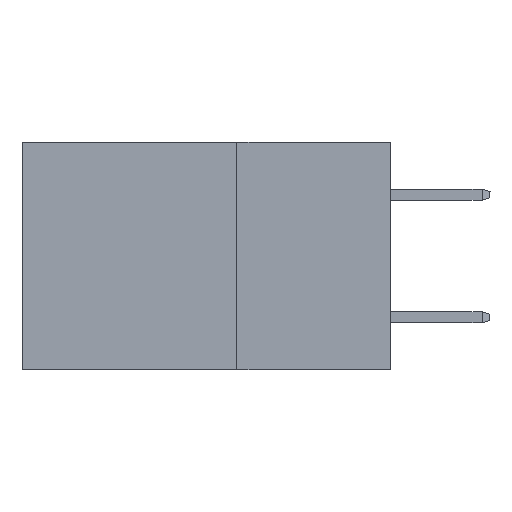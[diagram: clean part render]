
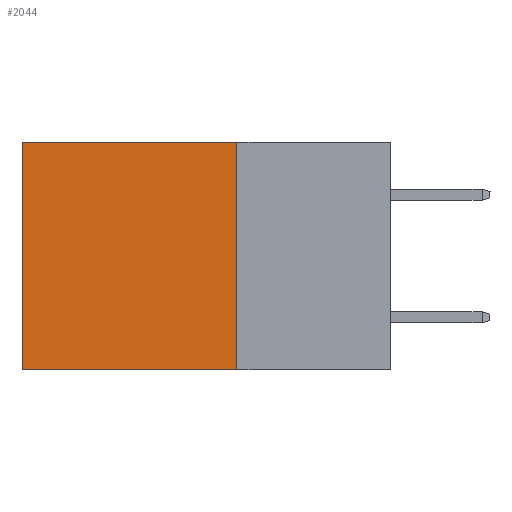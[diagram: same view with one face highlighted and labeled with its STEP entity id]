
A CAD part, left-side view. The second image highlights one B-rep face of the part: STEP entity #2044.
In plain terms, the highlighted planar face has unit normal (-1, 0, 0).
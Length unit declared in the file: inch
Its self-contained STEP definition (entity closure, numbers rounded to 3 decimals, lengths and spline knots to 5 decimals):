
#1630 = DIRECTION ( 'NONE',  ( 0., 1., 0. ) ) ;
#2005 = FACE_OUTER_BOUND ( 'NONE', #10825, .T. ) ;
#2044 = ADVANCED_FACE ( 'NONE', ( #2005 ), #17550, .F. ) ;
#2303 = VECTOR ( 'NONE', #1630, 39.37008 ) ;
#6398 = VECTOR ( 'NONE', #15519, 39.37008 ) ;
#6489 = CARTESIAN_POINT ( 'NONE',  ( 0.2875, 0.6, 0. ) ) ;
#6581 = LINE ( 'NONE', #12437, #2303 ) ;
#6946 = LINE ( 'NONE', #11987, #6398 ) ;
#6952 = DIRECTION ( 'NONE',  ( 0., 0., -1. ) ) ;
#10624 = ORIENTED_EDGE ( 'NONE', *, *, #14713, .T. ) ;
#10825 = EDGE_LOOP ( 'NONE', ( #21320, #17972, #13858, #10624 ) ) ;
#11648 = VECTOR ( 'NONE', #20529, 39.37008 ) ;
#11987 = CARTESIAN_POINT ( 'NONE',  ( 0.2875, 0.25, 0. ) ) ;
#12207 = LINE ( 'NONE', #18798, #11648 ) ;
#12398 = VERTEX_POINT ( 'NONE', #18010 ) ;
#12437 = CARTESIAN_POINT ( 'NONE',  ( 0.2875, 0.25, -0.37 ) ) ;
#12933 = DIRECTION ( 'NONE',  ( 0., 0., -1. ) ) ;
#13021 = LINE ( 'NONE', #21703, #21279 ) ;
#13337 = CARTESIAN_POINT ( 'NONE',  ( 0.2875, 0.25, 0. ) ) ;
#13858 = ORIENTED_EDGE ( 'NONE', *, *, #18443, .F. ) ;
#14713 = EDGE_CURVE ( 'NONE', #17749, #22465, #6946, .T. ) ;
#15519 = DIRECTION ( 'NONE',  ( 0., 1., 0. ) ) ;
#15844 = CARTESIAN_POINT ( 'NONE',  ( 0.2875, 0.25, 0. ) ) ;
#16215 = EDGE_CURVE ( 'NONE', #22465, #12398, #13021, .T. ) ;
#16424 = CARTESIAN_POINT ( 'NONE',  ( 0.2875, 0.25, -0.37 ) ) ;
#16731 = EDGE_CURVE ( 'NONE', #18204, #12398, #6581, .T. ) ;
#17550 = PLANE ( 'NONE',  #21333 ) ;
#17621 = DIRECTION ( 'NONE',  ( 1., 0., 0. ) ) ;
#17749 = VERTEX_POINT ( 'NONE', #13337 ) ;
#17972 = ORIENTED_EDGE ( 'NONE', *, *, #16731, .F. ) ;
#18010 = CARTESIAN_POINT ( 'NONE',  ( 0.2875, 0.6, -0.37 ) ) ;
#18204 = VERTEX_POINT ( 'NONE', #16424 ) ;
#18443 = EDGE_CURVE ( 'NONE', #17749, #18204, #12207, .T. ) ;
#18798 = CARTESIAN_POINT ( 'NONE',  ( 0.2875, 0.25, 0. ) ) ;
#20529 = DIRECTION ( 'NONE',  ( 0., 0., -1. ) ) ;
#21279 = VECTOR ( 'NONE', #12933, 39.37008 ) ;
#21320 = ORIENTED_EDGE ( 'NONE', *, *, #16215, .T. ) ;
#21333 = AXIS2_PLACEMENT_3D ( 'NONE', #15844, #17621, #6952 ) ;
#21703 = CARTESIAN_POINT ( 'NONE',  ( 0.2875, 0.6, 0. ) ) ;
#22465 = VERTEX_POINT ( 'NONE', #6489 ) ;
